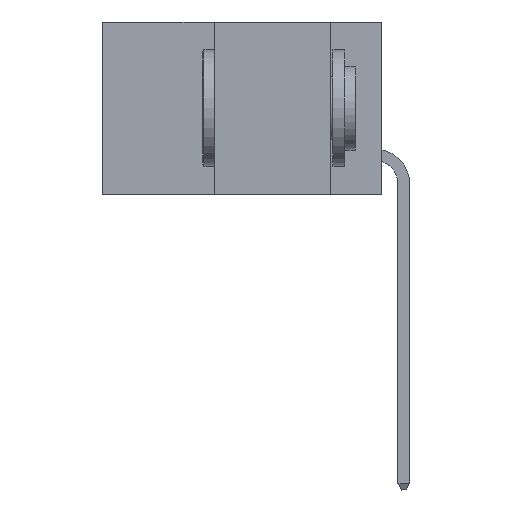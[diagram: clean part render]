
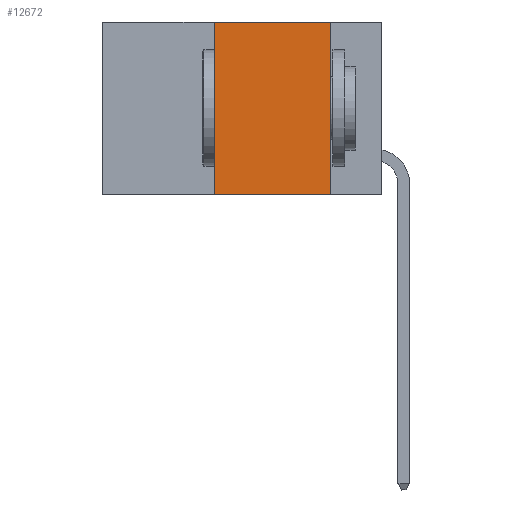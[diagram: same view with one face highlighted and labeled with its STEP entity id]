
A CAD part, left-side view. The second image highlights one B-rep face of the part: STEP entity #12672.
In plain terms, the highlighted planar face has unit normal (-1, 0, 0).
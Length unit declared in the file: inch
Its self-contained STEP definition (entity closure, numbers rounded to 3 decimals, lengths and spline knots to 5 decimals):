
#16 = DIRECTION ( 'NONE',  ( 1., 0., 0. ) ) ;
#551 = CARTESIAN_POINT ( 'NONE',  ( 0., 0.6, -0.37 ) ) ;
#679 = EDGE_CURVE ( 'NONE', #5648, #13150, #5006, .T. ) ;
#1816 = DIRECTION ( 'NONE',  ( 0., -1., 0. ) ) ;
#2098 = LINE ( 'NONE', #13875, #10947 ) ;
#2681 = CARTESIAN_POINT ( 'NONE',  ( 0., 0.11, 0. ) ) ;
#2949 = CARTESIAN_POINT ( 'NONE',  ( 0., 0.36, -0.37 ) ) ;
#2952 = AXIS2_PLACEMENT_3D ( 'NONE', #15487, #16, #14102 ) ;
#3178 = CARTESIAN_POINT ( 'NONE',  ( 0., 0.11, 0. ) ) ;
#4803 = ORIENTED_EDGE ( 'NONE', *, *, #9813, .F. ) ;
#5006 = LINE ( 'NONE', #15715, #14270 ) ;
#5429 = FACE_OUTER_BOUND ( 'NONE', #9050, .T. ) ;
#5454 = LINE ( 'NONE', #551, #9014 ) ;
#5648 = VERTEX_POINT ( 'NONE', #13487 ) ;
#6167 = LINE ( 'NONE', #2681, #12768 ) ;
#6438 = ORIENTED_EDGE ( 'NONE', *, *, #8031, .F. ) ;
#6460 = VERTEX_POINT ( 'NONE', #9937 ) ;
#7139 = ORIENTED_EDGE ( 'NONE', *, *, #679, .F. ) ;
#8031 = EDGE_CURVE ( 'NONE', #13150, #6460, #6167, .T. ) ;
#9014 = VECTOR ( 'NONE', #9242, 39.37008 ) ;
#9050 = EDGE_LOOP ( 'NONE', ( #6438, #7139, #4803, #18140 ) ) ;
#9109 = EDGE_CURVE ( 'NONE', #18266, #6460, #5454, .T. ) ;
#9242 = DIRECTION ( 'NONE',  ( 0., -1., 0. ) ) ;
#9813 = EDGE_CURVE ( 'NONE', #18266, #5648, #2098, .T. ) ;
#9937 = CARTESIAN_POINT ( 'NONE',  ( 0., 0.11, -0.37 ) ) ;
#10947 = VECTOR ( 'NONE', #11589, 39.37008 ) ;
#11589 = DIRECTION ( 'NONE',  ( 0., 0., 1. ) ) ;
#12672 = ADVANCED_FACE ( 'NONE', ( #5429 ), #14286, .F. ) ;
#12768 = VECTOR ( 'NONE', #16807, 39.37008 ) ;
#13150 = VERTEX_POINT ( 'NONE', #3178 ) ;
#13487 = CARTESIAN_POINT ( 'NONE',  ( 0., 0.36, 0. ) ) ;
#13875 = CARTESIAN_POINT ( 'NONE',  ( 0., 0.36, 0. ) ) ;
#14102 = DIRECTION ( 'NONE',  ( 0., 0., -1. ) ) ;
#14270 = VECTOR ( 'NONE', #1816, 39.37008 ) ;
#14286 = PLANE ( 'NONE',  #2952 ) ;
#15487 = CARTESIAN_POINT ( 'NONE',  ( 0., 0.6, 0. ) ) ;
#15715 = CARTESIAN_POINT ( 'NONE',  ( 0., 0.6, 0. ) ) ;
#16807 = DIRECTION ( 'NONE',  ( 0., 0., -1. ) ) ;
#18140 = ORIENTED_EDGE ( 'NONE', *, *, #9109, .T. ) ;
#18266 = VERTEX_POINT ( 'NONE', #2949 ) ;
